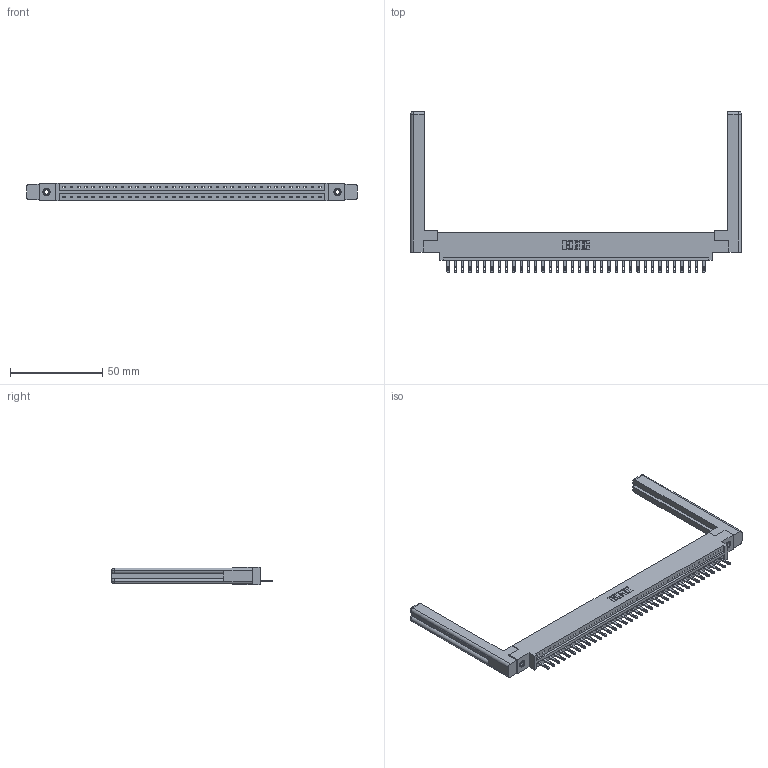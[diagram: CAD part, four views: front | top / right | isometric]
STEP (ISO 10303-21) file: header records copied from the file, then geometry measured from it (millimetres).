
FILE_DESCRIPTION (( 'STEP AP203' ), '1' );
FILE_NAME ('337-036-500-658.STEP', '2019-10-01T13:37:36', ( '' ), ( '' ), 'SwSTEP 2.0', 'SolidWorks 2016', '' );
FILE_SCHEMA (( 'CONFIG_CONTROL_DESIGN' ));
Length unit declared in the file: inch
Products named in the file (5): 345-250-001_345-250-001-102; 307-220-058; 345-292-001_345-293-100; 337 Part_0.170 Offset - 0.156 Dia-TI; 337-036-500-658
Assembly tree (41 placements, depth 2):
  337-036-500-658
    337 Part_0.170 Offset - 0.156 Dia-TI
    345-292-001_345-293-100  x36
    345-250-001_345-250-001-102  x2
    307-220-058  x2
Bounding box: 179.27 x 87.25 x 9.4 mm (x, y, z)
Volume: 25624.3 mm3; surface area: 24438.1 mm2
Topology: 41 solids, 41 shells, 2348 faces, 7157 edges, 4758 vertices
Faces by surface type: plane 1598, cylinder 726, cone 12, torus 12
Entity records: 30232 total; most frequent: CARTESIAN_POINT 5265, ORIENTED_EDGE 5176, DIRECTION 4464, EDGE_CURVE 2588, LINE 2408, VECTOR 2408, VERTEX_POINT 1718, AXIS2_PLACEMENT_3D 1028
